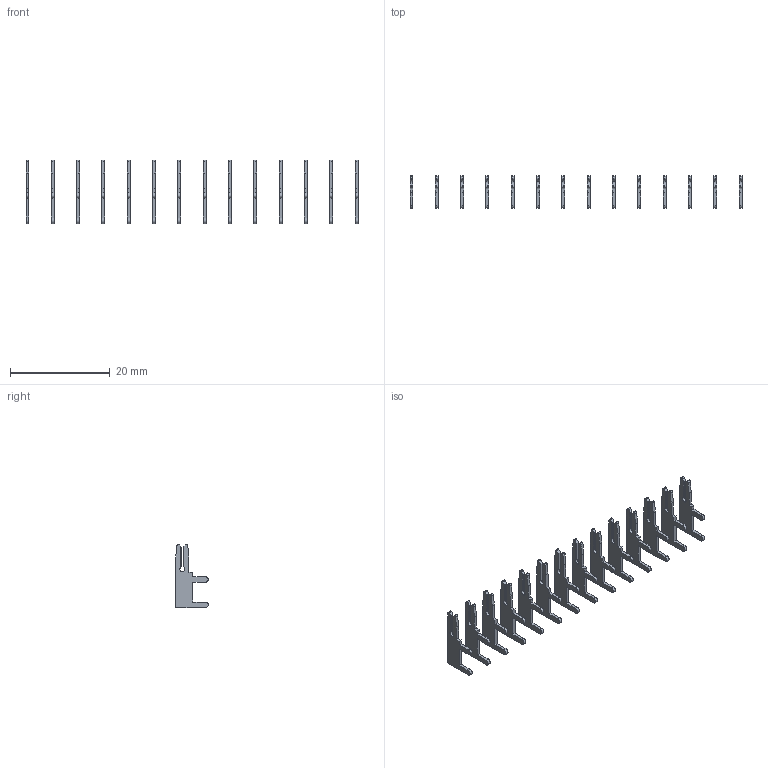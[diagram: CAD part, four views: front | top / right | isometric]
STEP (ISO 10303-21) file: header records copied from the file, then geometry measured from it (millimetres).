
FILE_DESCRIPTION (( 'STEP AP203' ), '1' );
FILE_NAME ('105-014-203-200.STEP', '2020-08-29T23:27:15', ( '' ), ( '' ), 'SwSTEP 2.0', 'SolidWorks 2020', '' );
FILE_SCHEMA (( 'CONFIG_CONTROL_DESIGN' ));
Length unit declared in the file: inch
Products named in the file (2): 105-014-203-200; 100-290-001_100-290-203
Assembly tree (14 placements, depth 2):
  105-014-203-200
    100-290-001_100-290-203  x14
Bounding box: 66.64 x 6.53 x 12.7 mm (x, y, z)
Volume: 353.4 mm3; surface area: 1620.1 mm2
Topology: 14 solids, 14 shells, 392 faces, 1092 edges, 728 vertices
Faces by surface type: plane 294, cylinder 98
Entity records: 1512 total; most frequent: CARTESIAN_POINT 187, DIRECTION 178, ORIENTED_EDGE 156, EDGE_CURVE 78, LINE 60, VECTOR 60, AXIS2_PLACEMENT_3D 59, VERTEX_POINT 52
